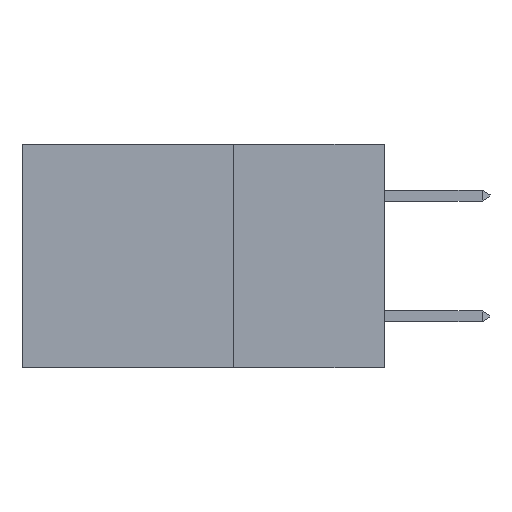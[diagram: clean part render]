
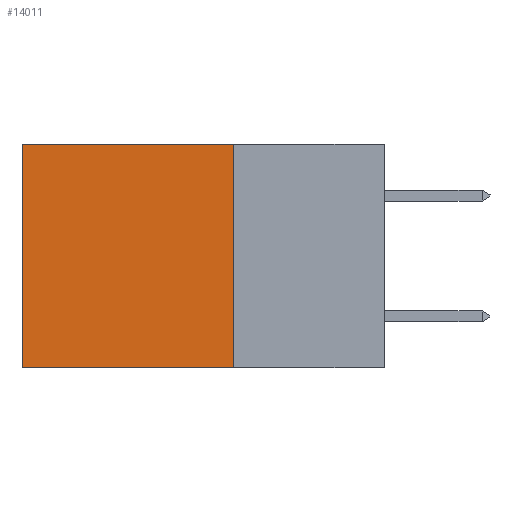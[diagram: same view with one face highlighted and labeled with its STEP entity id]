
A CAD part, left-side view. The second image highlights one B-rep face of the part: STEP entity #14011.
In plain terms, the highlighted planar face has unit normal (-1, 0, 0).
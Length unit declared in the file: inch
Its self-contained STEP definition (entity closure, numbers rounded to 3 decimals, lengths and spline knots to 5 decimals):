
#852 = ORIENTED_EDGE ( 'NONE', *, *, #3244, .T. ) ;
#957 = PLANE ( 'NONE',  #13642 ) ;
#991 = VERTEX_POINT ( 'NONE', #5233 ) ;
#1038 = CARTESIAN_POINT ( 'NONE',  ( 0.2875, 0.25, 0. ) ) ;
#1079 = VECTOR ( 'NONE', #12290, 39.37008 ) ;
#1599 = DIRECTION ( 'NONE',  ( 0., 1., 0. ) ) ;
#1982 = EDGE_CURVE ( 'NONE', #9243, #14928, #12374, .T. ) ;
#2331 = ORIENTED_EDGE ( 'NONE', *, *, #12930, .F. ) ;
#2369 = CARTESIAN_POINT ( 'NONE',  ( 0.2875, 0.25, -0.37 ) ) ;
#2372 = CARTESIAN_POINT ( 'NONE',  ( 0.2875, 0.6, 0. ) ) ;
#2664 = LINE ( 'NONE', #2753, #11462 ) ;
#2708 = CARTESIAN_POINT ( 'NONE',  ( 0.2875, 0.25, -0.37 ) ) ;
#2753 = CARTESIAN_POINT ( 'NONE',  ( 0.2875, 0.25, 0. ) ) ;
#2963 = CARTESIAN_POINT ( 'NONE',  ( 0.2875, 0.25, 0. ) ) ;
#3244 = EDGE_CURVE ( 'NONE', #11753, #14928, #7511, .T. ) ;
#4202 = LINE ( 'NONE', #2963, #12860 ) ;
#4665 = DIRECTION ( 'NONE',  ( 1., 0., 0. ) ) ;
#4818 = FACE_OUTER_BOUND ( 'NONE', #13788, .T. ) ;
#5233 = CARTESIAN_POINT ( 'NONE',  ( 0.2875, 0.25, 0. ) ) ;
#6163 = DIRECTION ( 'NONE',  ( 0., 0., -1. ) ) ;
#6199 = VECTOR ( 'NONE', #10042, 39.37008 ) ;
#7511 = LINE ( 'NONE', #2372, #6199 ) ;
#9243 = VERTEX_POINT ( 'NONE', #2708 ) ;
#9360 = EDGE_CURVE ( 'NONE', #991, #11753, #4202, .T. ) ;
#9980 = ORIENTED_EDGE ( 'NONE', *, *, #9360, .T. ) ;
#10042 = DIRECTION ( 'NONE',  ( 0., 0., -1. ) ) ;
#11462 = VECTOR ( 'NONE', #14676, 39.37008 ) ;
#11753 = VERTEX_POINT ( 'NONE', #14850 ) ;
#12290 = DIRECTION ( 'NONE',  ( 0., 1., 0. ) ) ;
#12374 = LINE ( 'NONE', #2369, #1079 ) ;
#12674 = CARTESIAN_POINT ( 'NONE',  ( 0.2875, 0.6, -0.37 ) ) ;
#12860 = VECTOR ( 'NONE', #1599, 39.37008 ) ;
#12930 = EDGE_CURVE ( 'NONE', #991, #9243, #2664, .T. ) ;
#13642 = AXIS2_PLACEMENT_3D ( 'NONE', #1038, #4665, #6163 ) ;
#13788 = EDGE_LOOP ( 'NONE', ( #852, #16218, #2331, #9980 ) ) ;
#14011 = ADVANCED_FACE ( 'NONE', ( #4818 ), #957, .F. ) ;
#14676 = DIRECTION ( 'NONE',  ( 0., 0., -1. ) ) ;
#14850 = CARTESIAN_POINT ( 'NONE',  ( 0.2875, 0.6, 0. ) ) ;
#14928 = VERTEX_POINT ( 'NONE', #12674 ) ;
#16218 = ORIENTED_EDGE ( 'NONE', *, *, #1982, .F. ) ;
